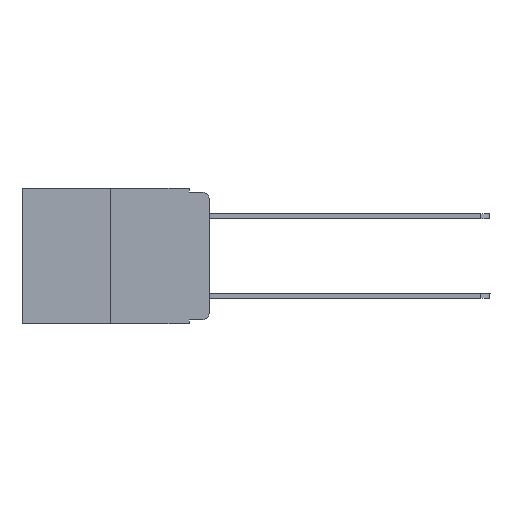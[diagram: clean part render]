
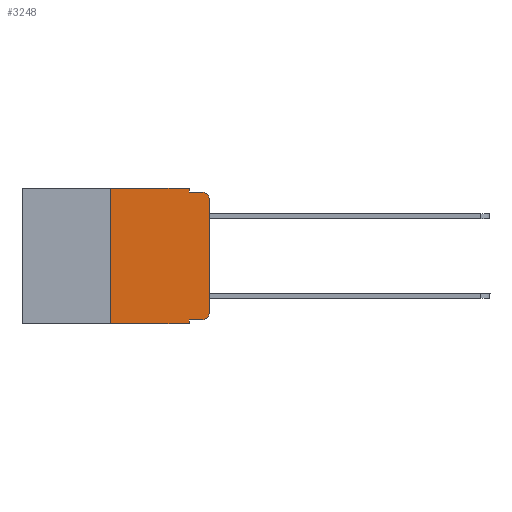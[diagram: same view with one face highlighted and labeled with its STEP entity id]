
A CAD part, left-side view. The second image highlights one B-rep face of the part: STEP entity #3248.
In plain terms, the highlighted planar face has unit normal (-1, 0, 0).
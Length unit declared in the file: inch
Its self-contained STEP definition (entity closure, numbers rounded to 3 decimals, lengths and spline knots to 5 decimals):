
#199 = VERTEX_POINT ( 'NONE', #17681 ) ;
#520 = ORIENTED_EDGE ( 'NONE', *, *, #5298, .F. ) ;
#858 = ORIENTED_EDGE ( 'NONE', *, *, #20106, .T. ) ;
#1192 = CARTESIAN_POINT ( 'NONE',  ( 0., 0.02, -0.01 ) ) ;
#1502 = CARTESIAN_POINT ( 'NONE',  ( 0., 0.051, -0.333 ) ) ;
#1504 = DIRECTION ( 'NONE',  ( 0., 0., 1. ) ) ;
#1750 = AXIS2_PLACEMENT_3D ( 'NONE', #10432, #16909, #17009 ) ;
#2019 = CARTESIAN_POINT ( 'NONE',  ( 0., 0.051, 0. ) ) ;
#2144 = LINE ( 'NONE', #16534, #3298 ) ;
#2235 = ORIENTED_EDGE ( 'NONE', *, *, #2934, .T. ) ;
#2369 = VECTOR ( 'NONE', #1504, 39.37008 ) ;
#2630 = CARTESIAN_POINT ( 'NONE',  ( 0., 0.25, 0. ) ) ;
#2635 = EDGE_CURVE ( 'NONE', #10678, #5390, #10397, .T. ) ;
#2681 = ORIENTED_EDGE ( 'NONE', *, *, #10437, .T. ) ;
#2934 = EDGE_CURVE ( 'NONE', #16387, #4414, #4705, .T. ) ;
#2988 = VECTOR ( 'NONE', #21173, 39.37008 ) ;
#3248 = ADVANCED_FACE ( 'NONE', ( #21232 ), #6478, .F. ) ;
#3298 = VECTOR ( 'NONE', #8556, 39.37008 ) ;
#4321 = DIRECTION ( 'NONE',  ( 0., 0., 1. ) ) ;
#4414 = VERTEX_POINT ( 'NONE', #13644 ) ;
#4705 = LINE ( 'NONE', #1502, #2988 ) ;
#5298 = EDGE_CURVE ( 'NONE', #10035, #15366, #12872, .T. ) ;
#5354 = LINE ( 'NONE', #19863, #20260 ) ;
#5368 = DIRECTION ( 'NONE',  ( 0., 0., -1. ) ) ;
#5390 = VERTEX_POINT ( 'NONE', #16635 ) ;
#5638 = LINE ( 'NONE', #13566, #13044 ) ;
#6009 = CARTESIAN_POINT ( 'NONE',  ( 0., 0.473, 0. ) ) ;
#6316 = CARTESIAN_POINT ( 'NONE',  ( 0., 0., -0.03 ) ) ;
#6378 = EDGE_CURVE ( 'NONE', #15366, #10678, #12554, .T. ) ;
#6478 = PLANE ( 'NONE',  #19619 ) ;
#6918 = VECTOR ( 'NONE', #5368, 39.37008 ) ;
#7292 = DIRECTION ( 'NONE',  ( 0., -1., 0. ) ) ;
#7388 = CARTESIAN_POINT ( 'NONE',  ( 0., 0.02, -0.03 ) ) ;
#7573 = EDGE_CURVE ( 'NONE', #5390, #18162, #2144, .T. ) ;
#8389 = ORIENTED_EDGE ( 'NONE', *, *, #19661, .T. ) ;
#8460 = ORIENTED_EDGE ( 'NONE', *, *, #13816, .F. ) ;
#8556 = DIRECTION ( 'NONE',  ( 0., -1., 0. ) ) ;
#8570 = ORIENTED_EDGE ( 'NONE', *, *, #14304, .T. ) ;
#8581 = CIRCLE ( 'NONE', #1750, 0.02 ) ;
#8826 = DIRECTION ( 'NONE',  ( 0., 0., -1. ) ) ;
#9538 = AXIS2_PLACEMENT_3D ( 'NONE', #7388, #14040, #12224 ) ;
#9712 = DIRECTION ( 'NONE',  ( 0., 0., -1. ) ) ;
#10035 = VERTEX_POINT ( 'NONE', #17737 ) ;
#10071 = CARTESIAN_POINT ( 'NONE',  ( 0., 0.051, 0. ) ) ;
#10397 = LINE ( 'NONE', #10071, #6918 ) ;
#10432 = CARTESIAN_POINT ( 'NONE',  ( 0., 0.02, -0.313 ) ) ;
#10437 = EDGE_CURVE ( 'NONE', #10460, #18162, #16064, .T. ) ;
#10460 = VERTEX_POINT ( 'NONE', #6316 ) ;
#10678 = VERTEX_POINT ( 'NONE', #2019 ) ;
#11555 = EDGE_LOOP ( 'NONE', ( #8570, #2681, #12216, #11999, #18581, #520, #8389, #8460, #2235, #858 ) ) ;
#11686 = VECTOR ( 'NONE', #4321, 39.37008 ) ;
#11815 = VECTOR ( 'NONE', #7292, 39.37008 ) ;
#11999 = ORIENTED_EDGE ( 'NONE', *, *, #2635, .F. ) ;
#12216 = ORIENTED_EDGE ( 'NONE', *, *, #7573, .F. ) ;
#12224 = DIRECTION ( 'NONE',  ( 0., 0., -1. ) ) ;
#12554 = LINE ( 'NONE', #6009, #11815 ) ;
#12872 = LINE ( 'NONE', #13080, #2369 ) ;
#13044 = VECTOR ( 'NONE', #8826, 39.37008 ) ;
#13080 = CARTESIAN_POINT ( 'NONE',  ( 0., 0.25, 0. ) ) ;
#13566 = CARTESIAN_POINT ( 'NONE',  ( 0., 0.051, 0. ) ) ;
#13644 = CARTESIAN_POINT ( 'NONE',  ( 0., 0.02, -0.333 ) ) ;
#13816 = EDGE_CURVE ( 'NONE', #16387, #199, #5638, .T. ) ;
#13860 = CARTESIAN_POINT ( 'NONE',  ( 0., 0., 0. ) ) ;
#14040 = DIRECTION ( 'NONE',  ( -1., 0., 0. ) ) ;
#14304 = EDGE_CURVE ( 'NONE', #18660, #10460, #15474, .T. ) ;
#15366 = VERTEX_POINT ( 'NONE', #2630 ) ;
#15474 = LINE ( 'NONE', #13860, #11686 ) ;
#16064 = CIRCLE ( 'NONE', #9538, 0.02 ) ;
#16387 = VERTEX_POINT ( 'NONE', #20991 ) ;
#16534 = CARTESIAN_POINT ( 'NONE',  ( 0., 0.051, -0.01 ) ) ;
#16635 = CARTESIAN_POINT ( 'NONE',  ( 0., 0.051, -0.01 ) ) ;
#16742 = DIRECTION ( 'NONE',  ( 0., -1., 0. ) ) ;
#16909 = DIRECTION ( 'NONE',  ( -1., 0., 0. ) ) ;
#17009 = DIRECTION ( 'NONE',  ( 0., 0., -1. ) ) ;
#17681 = CARTESIAN_POINT ( 'NONE',  ( 0., 0.051, -0.343 ) ) ;
#17737 = CARTESIAN_POINT ( 'NONE',  ( 0., 0.25, -0.343 ) ) ;
#18000 = DIRECTION ( 'NONE',  ( 1., 0., 0. ) ) ;
#18162 = VERTEX_POINT ( 'NONE', #1192 ) ;
#18581 = ORIENTED_EDGE ( 'NONE', *, *, #6378, .F. ) ;
#18660 = VERTEX_POINT ( 'NONE', #20724 ) ;
#19406 = CARTESIAN_POINT ( 'NONE',  ( 0., 0.473, 0. ) ) ;
#19619 = AXIS2_PLACEMENT_3D ( 'NONE', #19406, #18000, #9712 ) ;
#19661 = EDGE_CURVE ( 'NONE', #10035, #199, #5354, .T. ) ;
#19863 = CARTESIAN_POINT ( 'NONE',  ( 0., 0.473, -0.343 ) ) ;
#20106 = EDGE_CURVE ( 'NONE', #4414, #18660, #8581, .T. ) ;
#20260 = VECTOR ( 'NONE', #16742, 39.37008 ) ;
#20724 = CARTESIAN_POINT ( 'NONE',  ( 0., 0., -0.313 ) ) ;
#20991 = CARTESIAN_POINT ( 'NONE',  ( 0., 0.051, -0.333 ) ) ;
#21173 = DIRECTION ( 'NONE',  ( 0., -1., 0. ) ) ;
#21232 = FACE_OUTER_BOUND ( 'NONE', #11555, .T. ) ;
